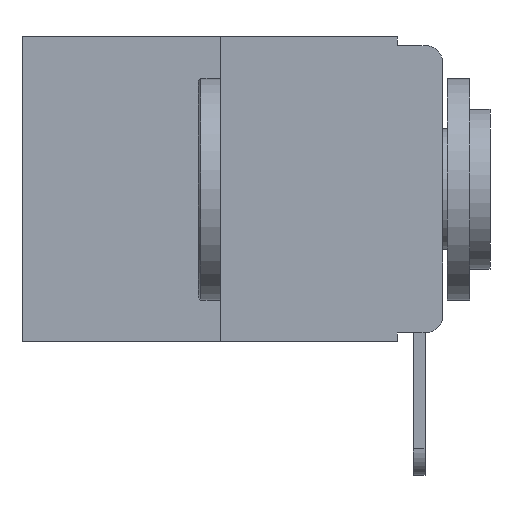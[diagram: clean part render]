
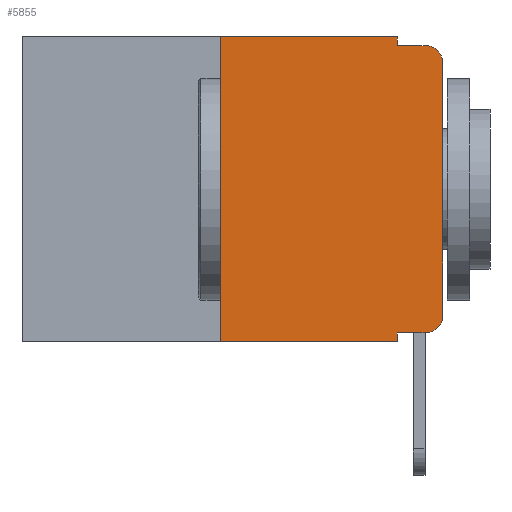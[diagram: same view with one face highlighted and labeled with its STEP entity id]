
A CAD part, left-side view. The second image highlights one B-rep face of the part: STEP entity #5855.
In plain terms, the highlighted planar face has unit normal (-1, 0, 0).
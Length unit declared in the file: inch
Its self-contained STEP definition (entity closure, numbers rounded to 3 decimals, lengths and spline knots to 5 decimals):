
#283 = ORIENTED_EDGE ( 'NONE', *, *, #421, .F. ) ;
#319 = ORIENTED_EDGE ( 'NONE', *, *, #8012, .F. ) ;
#323 = VECTOR ( 'NONE', #6099, 39.37008 ) ;
#421 = EDGE_CURVE ( 'NONE', #8217, #1417, #13044, .T. ) ;
#476 = ORIENTED_EDGE ( 'NONE', *, *, #11268, .F. ) ;
#533 = DIRECTION ( 'NONE',  ( 0., 0., -1. ) ) ;
#718 = ORIENTED_EDGE ( 'NONE', *, *, #6189, .T. ) ;
#760 = ORIENTED_EDGE ( 'NONE', *, *, #5897, .F. ) ;
#891 = ORIENTED_EDGE ( 'NONE', *, *, #5186, .T. ) ;
#971 = EDGE_CURVE ( 'NONE', #4538, #2238, #13030, .T. ) ;
#1093 = ORIENTED_EDGE ( 'NONE', *, *, #5011, .T. ) ;
#1109 = VERTEX_POINT ( 'NONE', #11729 ) ;
#1268 = LINE ( 'NONE', #13563, #7294 ) ;
#1269 = DIRECTION ( 'NONE',  ( 0., -1., 0. ) ) ;
#1417 = VERTEX_POINT ( 'NONE', #5459 ) ;
#2238 = VERTEX_POINT ( 'NONE', #13316 ) ;
#2239 = CARTESIAN_POINT ( 'NONE',  ( 0., 0.02, -0.333 ) ) ;
#3294 = VERTEX_POINT ( 'NONE', #2239 ) ;
#3535 = LINE ( 'NONE', #5016, #323 ) ;
#3564 = DIRECTION ( 'NONE',  ( -1., 0., 0. ) ) ;
#3629 = CARTESIAN_POINT ( 'NONE',  ( 0., 0.473, -0.343 ) ) ;
#3935 = VECTOR ( 'NONE', #6031, 39.37008 ) ;
#4036 = DIRECTION ( 'NONE',  ( 0., 0., -1. ) ) ;
#4086 = CARTESIAN_POINT ( 'NONE',  ( 0., 0.051, 0. ) ) ;
#4516 = CARTESIAN_POINT ( 'NONE',  ( 0., 0., -0.313 ) ) ;
#4538 = VERTEX_POINT ( 'NONE', #4516 ) ;
#4685 = CARTESIAN_POINT ( 'NONE',  ( 0., 0.051, -0.01 ) ) ;
#4939 = CARTESIAN_POINT ( 'NONE',  ( 0., 0.051, 0. ) ) ;
#5011 = EDGE_CURVE ( 'NONE', #3294, #4538, #7125, .T. ) ;
#5016 = CARTESIAN_POINT ( 'NONE',  ( 0., 0.051, -0.01 ) ) ;
#5186 = EDGE_CURVE ( 'NONE', #11501, #3294, #1268, .T. ) ;
#5247 = VECTOR ( 'NONE', #1269, 39.37008 ) ;
#5256 = AXIS2_PLACEMENT_3D ( 'NONE', #9818, #3564, #10784 ) ;
#5389 = DIRECTION ( 'NONE',  ( 0., 0., 1. ) ) ;
#5402 = ORIENTED_EDGE ( 'NONE', *, *, #9336, .F. ) ;
#5442 = VERTEX_POINT ( 'NONE', #9177 ) ;
#5459 = CARTESIAN_POINT ( 'NONE',  ( 0., 0.051, 0. ) ) ;
#5481 = VECTOR ( 'NONE', #5389, 39.37008 ) ;
#5855 = ADVANCED_FACE ( 'NONE', ( #9300 ), #9260, .F. ) ;
#5897 = EDGE_CURVE ( 'NONE', #11501, #1109, #8996, .T. ) ;
#6031 = DIRECTION ( 'NONE',  ( 0., 0., -1. ) ) ;
#6099 = DIRECTION ( 'NONE',  ( 0., -1., 0. ) ) ;
#6189 = EDGE_CURVE ( 'NONE', #11504, #1109, #10935, .T. ) ;
#6304 = DIRECTION ( 'NONE',  ( 0., 0., -1. ) ) ;
#6386 = ORIENTED_EDGE ( 'NONE', *, *, #971, .T. ) ;
#6529 = DIRECTION ( 'NONE',  ( 0., 0., 1. ) ) ;
#7125 = CIRCLE ( 'NONE', #7296, 0.02 ) ;
#7272 = CARTESIAN_POINT ( 'NONE',  ( 0., 0.473, 0. ) ) ;
#7294 = VECTOR ( 'NONE', #11091, 39.37008 ) ;
#7296 = AXIS2_PLACEMENT_3D ( 'NONE', #10485, #10467, #6304 ) ;
#7587 = CARTESIAN_POINT ( 'NONE',  ( 0., 0., 0. ) ) ;
#7754 = EDGE_LOOP ( 'NONE', ( #6386, #12561, #476, #5402, #283, #319, #718, #760, #891, #1093 ) ) ;
#8012 = EDGE_CURVE ( 'NONE', #11504, #8217, #11898, .T. ) ;
#8217 = VERTEX_POINT ( 'NONE', #11771 ) ;
#8996 = LINE ( 'NONE', #4086, #11252 ) ;
#9177 = CARTESIAN_POINT ( 'NONE',  ( 0., 0.02, -0.01 ) ) ;
#9260 = PLANE ( 'NONE',  #12754 ) ;
#9300 = FACE_OUTER_BOUND ( 'NONE', #7754, .T. ) ;
#9311 = CARTESIAN_POINT ( 'NONE',  ( 0., 0.473, 0. ) ) ;
#9336 = EDGE_CURVE ( 'NONE', #1417, #10053, #12028, .T. ) ;
#9379 = VECTOR ( 'NONE', #6529, 39.37008 ) ;
#9818 = CARTESIAN_POINT ( 'NONE',  ( 0., 0.02, -0.03 ) ) ;
#10053 = VERTEX_POINT ( 'NONE', #4685 ) ;
#10228 = DIRECTION ( 'NONE',  ( 1., 0., 0. ) ) ;
#10316 = CARTESIAN_POINT ( 'NONE',  ( 0., 0.051, -0.333 ) ) ;
#10467 = DIRECTION ( 'NONE',  ( -1., 0., 0. ) ) ;
#10485 = CARTESIAN_POINT ( 'NONE',  ( 0., 0.02, -0.313 ) ) ;
#10491 = CARTESIAN_POINT ( 'NONE',  ( 0., 0.25, 0. ) ) ;
#10562 = VECTOR ( 'NONE', #10954, 39.37008 ) ;
#10784 = DIRECTION ( 'NONE',  ( 0., 0., -1. ) ) ;
#10935 = LINE ( 'NONE', #3629, #5247 ) ;
#10954 = DIRECTION ( 'NONE',  ( 0., -1., 0. ) ) ;
#11091 = DIRECTION ( 'NONE',  ( 0., -1., 0. ) ) ;
#11252 = VECTOR ( 'NONE', #533, 39.37008 ) ;
#11268 = EDGE_CURVE ( 'NONE', #10053, #5442, #3535, .T. ) ;
#11501 = VERTEX_POINT ( 'NONE', #10316 ) ;
#11504 = VERTEX_POINT ( 'NONE', #13148 ) ;
#11729 = CARTESIAN_POINT ( 'NONE',  ( 0., 0.051, -0.343 ) ) ;
#11771 = CARTESIAN_POINT ( 'NONE',  ( 0., 0.25, 0. ) ) ;
#11898 = LINE ( 'NONE', #10491, #9379 ) ;
#11976 = CIRCLE ( 'NONE', #5256, 0.02 ) ;
#12028 = LINE ( 'NONE', #4939, #3935 ) ;
#12561 = ORIENTED_EDGE ( 'NONE', *, *, #13122, .T. ) ;
#12754 = AXIS2_PLACEMENT_3D ( 'NONE', #7272, #10228, #4036 ) ;
#13030 = LINE ( 'NONE', #7587, #5481 ) ;
#13044 = LINE ( 'NONE', #9311, #10562 ) ;
#13122 = EDGE_CURVE ( 'NONE', #2238, #5442, #11976, .T. ) ;
#13148 = CARTESIAN_POINT ( 'NONE',  ( 0., 0.25, -0.343 ) ) ;
#13316 = CARTESIAN_POINT ( 'NONE',  ( 0., 0., -0.03 ) ) ;
#13563 = CARTESIAN_POINT ( 'NONE',  ( 0., 0.051, -0.333 ) ) ;
